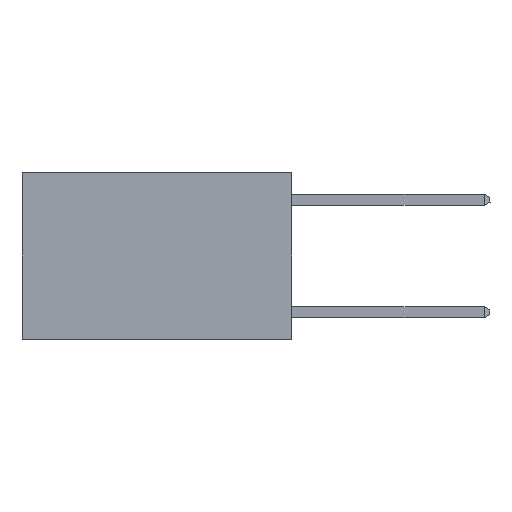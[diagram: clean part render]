
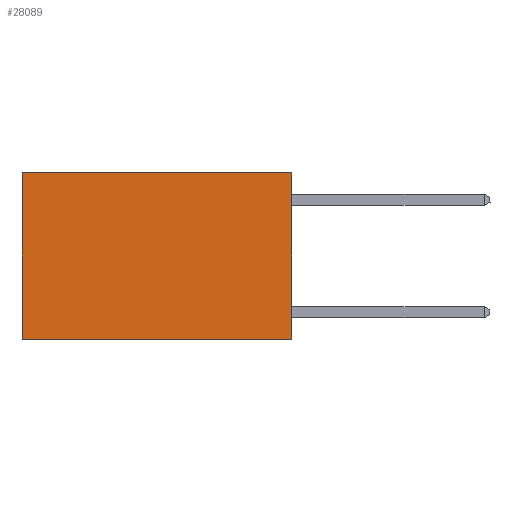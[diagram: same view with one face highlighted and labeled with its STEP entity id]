
A CAD part, left-side view. The second image highlights one B-rep face of the part: STEP entity #28089.
In plain terms, the highlighted planar face has unit normal (-1, 0, 0).
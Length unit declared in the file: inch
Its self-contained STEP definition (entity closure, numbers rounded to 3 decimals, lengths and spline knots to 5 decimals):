
#830 = EDGE_CURVE ( 'NONE', #15227, #19425, #26694, .T. ) ;
#1542 = ORIENTED_EDGE ( 'NONE', *, *, #18118, .F. ) ;
#1771 = CARTESIAN_POINT ( 'NONE',  ( 0.2625, 0., 0. ) ) ;
#3867 = VECTOR ( 'NONE', #16242, 39.37008 ) ;
#3937 = ORIENTED_EDGE ( 'NONE', *, *, #26933, .T. ) ;
#6416 = DIRECTION ( 'NONE',  ( 0., 0., -1. ) ) ;
#8839 = VECTOR ( 'NONE', #17323, 39.37008 ) ;
#9954 = LINE ( 'NONE', #27875, #8839 ) ;
#11467 = VERTEX_POINT ( 'NONE', #14433 ) ;
#11582 = DIRECTION ( 'NONE',  ( 0., 0., -1. ) ) ;
#12311 = CARTESIAN_POINT ( 'NONE',  ( 0.2625, 0., 0. ) ) ;
#12397 = VERTEX_POINT ( 'NONE', #14660 ) ;
#12496 = AXIS2_PLACEMENT_3D ( 'NONE', #1771, #18324, #11582 ) ;
#13165 = EDGE_CURVE ( 'NONE', #15227, #11467, #16298, .T. ) ;
#14433 = CARTESIAN_POINT ( 'NONE',  ( 0.2625, 0.6, 0. ) ) ;
#14660 = CARTESIAN_POINT ( 'NONE',  ( 0.2625, 0.6, -0.37 ) ) ;
#15227 = VERTEX_POINT ( 'NONE', #24623 ) ;
#16242 = DIRECTION ( 'NONE',  ( 0., 1., 0. ) ) ;
#16298 = LINE ( 'NONE', #28886, #20729 ) ;
#16833 = VECTOR ( 'NONE', #6416, 39.37008 ) ;
#17323 = DIRECTION ( 'NONE',  ( 0., 0., -1. ) ) ;
#18118 = EDGE_CURVE ( 'NONE', #19425, #12397, #21073, .T. ) ;
#18324 = DIRECTION ( 'NONE',  ( 1., 0., 0. ) ) ;
#19425 = VERTEX_POINT ( 'NONE', #19481 ) ;
#19481 = CARTESIAN_POINT ( 'NONE',  ( 0.2625, 0., -0.37 ) ) ;
#20729 = VECTOR ( 'NONE', #28974, 39.37008 ) ;
#21073 = LINE ( 'NONE', #25556, #3867 ) ;
#22258 = ORIENTED_EDGE ( 'NONE', *, *, #830, .F. ) ;
#23060 = FACE_OUTER_BOUND ( 'NONE', #29576, .T. ) ;
#24623 = CARTESIAN_POINT ( 'NONE',  ( 0.2625, 0., 0. ) ) ;
#25556 = CARTESIAN_POINT ( 'NONE',  ( 0.2625, 0., -0.37 ) ) ;
#26694 = LINE ( 'NONE', #12311, #16833 ) ;
#26933 = EDGE_CURVE ( 'NONE', #11467, #12397, #9954, .T. ) ;
#27875 = CARTESIAN_POINT ( 'NONE',  ( 0.2625, 0.6, 0. ) ) ;
#28043 = ORIENTED_EDGE ( 'NONE', *, *, #13165, .T. ) ;
#28089 = ADVANCED_FACE ( 'NONE', ( #23060 ), #29792, .F. ) ;
#28886 = CARTESIAN_POINT ( 'NONE',  ( 0.2625, 0., 0. ) ) ;
#28974 = DIRECTION ( 'NONE',  ( 0., 1., 0. ) ) ;
#29576 = EDGE_LOOP ( 'NONE', ( #3937, #1542, #22258, #28043 ) ) ;
#29792 = PLANE ( 'NONE',  #12496 ) ;
